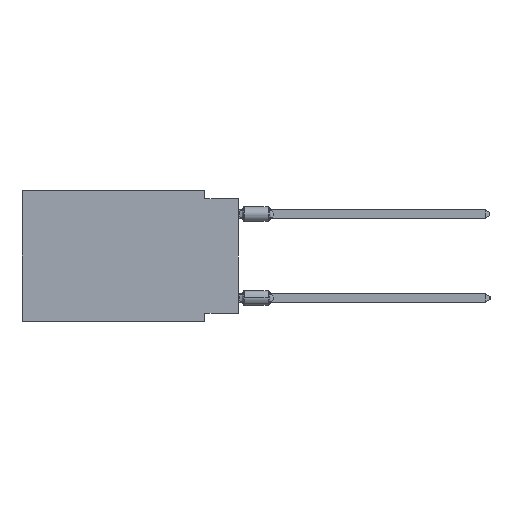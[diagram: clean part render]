
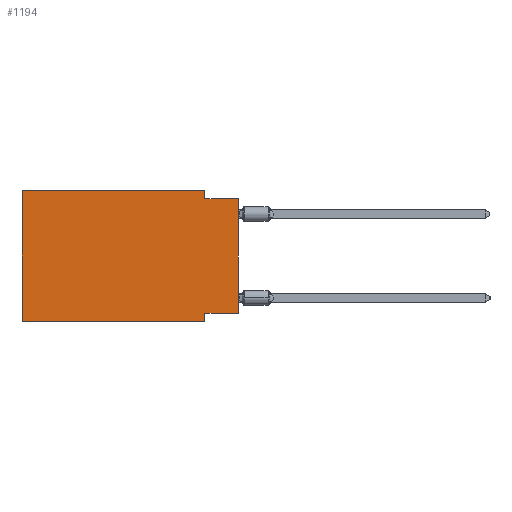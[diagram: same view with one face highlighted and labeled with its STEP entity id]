
A CAD part, left-side view. The second image highlights one B-rep face of the part: STEP entity #1194.
In plain terms, the highlighted planar face has unit normal (-1, 0, 0).
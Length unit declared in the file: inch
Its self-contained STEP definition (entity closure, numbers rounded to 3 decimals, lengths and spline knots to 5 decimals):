
#1194 = ADVANCED_FACE ( 'NONE', ( #38858 ), #34377, .F. ) ;
#1578 = CARTESIAN_POINT ( 'NONE',  ( 0., 0.1, -0.365 ) ) ;
#1622 = AXIS2_PLACEMENT_3D ( 'NONE', #52644, #11587, #7059 ) ;
#2901 = CARTESIAN_POINT ( 'NONE',  ( 0., 0., -0.025 ) ) ;
#3508 = ORIENTED_EDGE ( 'NONE', *, *, #21167, .F. ) ;
#3615 = VECTOR ( 'NONE', #4643, 39.37008 ) ;
#3653 = VECTOR ( 'NONE', #49616, 39.37008 ) ;
#3805 = VERTEX_POINT ( 'NONE', #2901 ) ;
#3902 = LINE ( 'NONE', #13764, #8860 ) ;
#4643 = DIRECTION ( 'NONE',  ( 0., -1., 0. ) ) ;
#5121 = LINE ( 'NONE', #32445, #31082 ) ;
#7059 = DIRECTION ( 'NONE',  ( 0., 0., -1. ) ) ;
#7764 = ORIENTED_EDGE ( 'NONE', *, *, #25870, .F. ) ;
#8014 = EDGE_CURVE ( 'NONE', #9779, #3805, #5121, .T. ) ;
#8370 = ORIENTED_EDGE ( 'NONE', *, *, #8014, .T. ) ;
#8860 = VECTOR ( 'NONE', #8961, 39.37008 ) ;
#8961 = DIRECTION ( 'NONE',  ( 0., -1., 0. ) ) ;
#9779 = VERTEX_POINT ( 'NONE', #29040 ) ;
#10727 = ORIENTED_EDGE ( 'NONE', *, *, #30193, .F. ) ;
#11587 = DIRECTION ( 'NONE',  ( 1., 0., 0. ) ) ;
#12199 = DIRECTION ( 'NONE',  ( 0., 0., -1. ) ) ;
#12320 = ORIENTED_EDGE ( 'NONE', *, *, #15587, .F. ) ;
#12448 = CARTESIAN_POINT ( 'NONE',  ( 0., 0.1, -0.025 ) ) ;
#13764 = CARTESIAN_POINT ( 'NONE',  ( 0., 0., -0.025 ) ) ;
#13832 = DIRECTION ( 'NONE',  ( 0., 0., 1. ) ) ;
#14523 = DIRECTION ( 'NONE',  ( 0., 1., 0. ) ) ;
#15587 = EDGE_CURVE ( 'NONE', #17511, #36955, #25697, .T. ) ;
#16666 = CARTESIAN_POINT ( 'NONE',  ( 0., 0.1, 0. ) ) ;
#17511 = VERTEX_POINT ( 'NONE', #51645 ) ;
#19027 = LINE ( 'NONE', #50500, #33633 ) ;
#19055 = CARTESIAN_POINT ( 'NONE',  ( 0., 0.1, -0.39 ) ) ;
#19699 = VECTOR ( 'NONE', #34541, 39.37008 ) ;
#20924 = ORIENTED_EDGE ( 'NONE', *, *, #42473, .F. ) ;
#21167 = EDGE_CURVE ( 'NONE', #42532, #17511, #41214, .T. ) ;
#22315 = LINE ( 'NONE', #40319, #3653 ) ;
#23073 = EDGE_LOOP ( 'NONE', ( #8370, #7764, #12320, #3508, #20924, #24848, #23171, #10727 ) ) ;
#23171 = ORIENTED_EDGE ( 'NONE', *, *, #55635, .F. ) ;
#24848 = ORIENTED_EDGE ( 'NONE', *, *, #51139, .T. ) ;
#25697 = LINE ( 'NONE', #16666, #32080 ) ;
#25870 = EDGE_CURVE ( 'NONE', #36955, #3805, #3902, .T. ) ;
#28352 = LINE ( 'NONE', #51722, #45540 ) ;
#29040 = CARTESIAN_POINT ( 'NONE',  ( 0., 0., -0.365 ) ) ;
#29235 = CARTESIAN_POINT ( 'NONE',  ( 0., 0.645, 0. ) ) ;
#30193 = EDGE_CURVE ( 'NONE', #9779, #33511, #19027, .T. ) ;
#31082 = VECTOR ( 'NONE', #13832, 39.37008 ) ;
#32080 = VECTOR ( 'NONE', #12199, 39.37008 ) ;
#32445 = CARTESIAN_POINT ( 'NONE',  ( 0., 0., 0. ) ) ;
#33511 = VERTEX_POINT ( 'NONE', #1578 ) ;
#33633 = VECTOR ( 'NONE', #14523, 39.37008 ) ;
#34377 = PLANE ( 'NONE',  #1622 ) ;
#34541 = DIRECTION ( 'NONE',  ( 0., 0., -1. ) ) ;
#36955 = VERTEX_POINT ( 'NONE', #12448 ) ;
#38858 = FACE_OUTER_BOUND ( 'NONE', #23073, .T. ) ;
#38923 = VERTEX_POINT ( 'NONE', #51311 ) ;
#40319 = CARTESIAN_POINT ( 'NONE',  ( 0., 0.645, -0.39 ) ) ;
#40810 = VERTEX_POINT ( 'NONE', #19055 ) ;
#41214 = LINE ( 'NONE', #59179, #3615 ) ;
#42473 = EDGE_CURVE ( 'NONE', #38923, #42532, #28352, .T. ) ;
#42532 = VERTEX_POINT ( 'NONE', #29235 ) ;
#44126 = CARTESIAN_POINT ( 'NONE',  ( 0., 0.1, -0.39 ) ) ;
#45540 = VECTOR ( 'NONE', #46641, 39.37008 ) ;
#46641 = DIRECTION ( 'NONE',  ( 0., 0., 1. ) ) ;
#49616 = DIRECTION ( 'NONE',  ( 0., -1., 0. ) ) ;
#50500 = CARTESIAN_POINT ( 'NONE',  ( 0., 0., -0.365 ) ) ;
#51139 = EDGE_CURVE ( 'NONE', #38923, #40810, #22315, .T. ) ;
#51311 = CARTESIAN_POINT ( 'NONE',  ( 0., 0.645, -0.39 ) ) ;
#51645 = CARTESIAN_POINT ( 'NONE',  ( 0., 0.1, 0. ) ) ;
#51722 = CARTESIAN_POINT ( 'NONE',  ( 0., 0.645, 0. ) ) ;
#52644 = CARTESIAN_POINT ( 'NONE',  ( 0., 0.645, 0. ) ) ;
#52803 = LINE ( 'NONE', #44126, #19699 ) ;
#55635 = EDGE_CURVE ( 'NONE', #33511, #40810, #52803, .T. ) ;
#59179 = CARTESIAN_POINT ( 'NONE',  ( 0., 0.645, 0. ) ) ;
